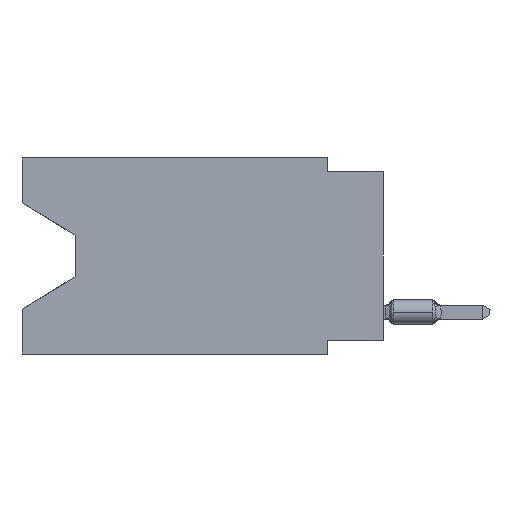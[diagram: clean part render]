
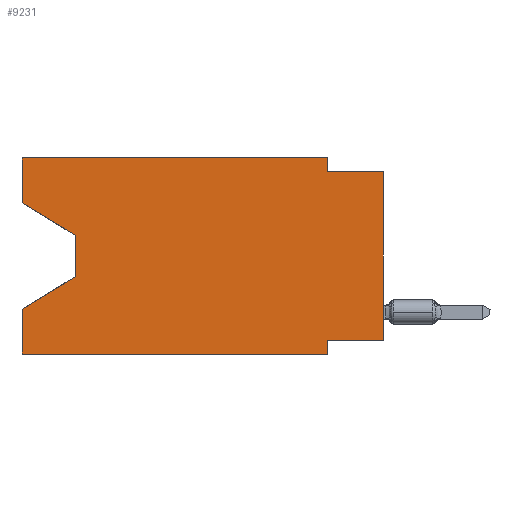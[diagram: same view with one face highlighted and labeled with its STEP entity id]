
A CAD part, left-side view. The second image highlights one B-rep face of the part: STEP entity #9231.
In plain terms, the highlighted planar face has unit normal (-1, 0, 0).
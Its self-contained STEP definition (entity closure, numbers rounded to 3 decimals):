
#89 = DIRECTION ( 'NONE',  ( 0., -0.855, -0.519 ) ) ;
#233 = CARTESIAN_POINT ( 'NONE',  ( 0., 16.383, 0. ) ) ;
#624 = ORIENTED_EDGE ( 'NONE', *, *, #20183, .T. ) ;
#1075 = ORIENTED_EDGE ( 'NONE', *, *, #25123, .T. ) ;
#1154 = CARTESIAN_POINT ( 'NONE',  ( 0., 16.383, 0. ) ) ;
#2207 = EDGE_CURVE ( 'NONE', #17085, #7352, #25438, .T. ) ;
#2250 = EDGE_CURVE ( 'NONE', #11897, #16530, #12424, .T. ) ;
#2312 = CARTESIAN_POINT ( 'NONE',  ( 0., 13.97, -5.385 ) ) ;
#2490 = PLANE ( 'NONE',  #31888 ) ;
#2529 = VECTOR ( 'NONE', #15556, 1000. ) ;
#3040 = EDGE_CURVE ( 'NONE', #7210, #9393, #24989, .T. ) ;
#3140 = VERTEX_POINT ( 'NONE', #23352 ) ;
#3518 = EDGE_CURVE ( 'NONE', #7352, #16530, #30788, .T. ) ;
#3834 = CARTESIAN_POINT ( 'NONE',  ( 0., 0., -8.255 ) ) ;
#4276 = ORIENTED_EDGE ( 'NONE', *, *, #25772, .F. ) ;
#4380 = LINE ( 'NONE', #15227, #20612 ) ;
#4514 = VECTOR ( 'NONE', #32102, 1000. ) ;
#4566 = LINE ( 'NONE', #23581, #4514 ) ;
#4785 = VECTOR ( 'NONE', #17779, 1000. ) ;
#5149 = DIRECTION ( 'NONE',  ( 1., 0., 0. ) ) ;
#5210 = VERTEX_POINT ( 'NONE', #28147 ) ;
#5321 = CARTESIAN_POINT ( 'NONE',  ( 0., 16.383, 0. ) ) ;
#6059 = CARTESIAN_POINT ( 'NONE',  ( 0., 2.54, -0.635 ) ) ;
#6115 = VECTOR ( 'NONE', #89, 1000. ) ;
#6906 = CARTESIAN_POINT ( 'NONE',  ( 0., 2.54, -8.89 ) ) ;
#7210 = VERTEX_POINT ( 'NONE', #2312 ) ;
#7352 = VERTEX_POINT ( 'NONE', #22215 ) ;
#7535 = LINE ( 'NONE', #32271, #6115 ) ;
#7767 = CARTESIAN_POINT ( 'NONE',  ( 0., 0., -0.635 ) ) ;
#8095 = EDGE_CURVE ( 'NONE', #17085, #34707, #4380, .T. ) ;
#8875 = VECTOR ( 'NONE', #14581, 1000. ) ;
#9231 = ADVANCED_FACE ( 'NONE', ( #29511 ), #2490, .F. ) ;
#9393 = VERTEX_POINT ( 'NONE', #30914 ) ;
#9701 = VERTEX_POINT ( 'NONE', #1154 ) ;
#9958 = VECTOR ( 'NONE', #24852, 1000. ) ;
#10152 = DIRECTION ( 'NONE',  ( 0., 0., -1. ) ) ;
#10633 = CARTESIAN_POINT ( 'NONE',  ( 0., 2.54, -8.89 ) ) ;
#10698 = ORIENTED_EDGE ( 'NONE', *, *, #22738, .F. ) ;
#11897 = VERTEX_POINT ( 'NONE', #25189 ) ;
#12424 = LINE ( 'NONE', #33763, #8875 ) ;
#14377 = ORIENTED_EDGE ( 'NONE', *, *, #33634, .F. ) ;
#14581 = DIRECTION ( 'NONE',  ( 0., -1., 0. ) ) ;
#14922 = CARTESIAN_POINT ( 'NONE',  ( 0., 0., -8.255 ) ) ;
#15227 = CARTESIAN_POINT ( 'NONE',  ( 0., 0., 0. ) ) ;
#15247 = ORIENTED_EDGE ( 'NONE', *, *, #3040, .T. ) ;
#15556 = DIRECTION ( 'NONE',  ( 0., 0., 1. ) ) ;
#15677 = LINE ( 'NONE', #24022, #20186 ) ;
#16282 = CARTESIAN_POINT ( 'NONE',  ( 0., 2.54, 0. ) ) ;
#16530 = VERTEX_POINT ( 'NONE', #10633 ) ;
#16658 = LINE ( 'NONE', #21818, #9958 ) ;
#17085 = VERTEX_POINT ( 'NONE', #3834 ) ;
#17779 = DIRECTION ( 'NONE',  ( 0., 0., -1. ) ) ;
#19285 = LINE ( 'NONE', #233, #31623 ) ;
#19436 = EDGE_LOOP ( 'NONE', ( #1075, #624, #15247, #10698, #22197, #28605, #26806, #34884, #4276, #21616, #14377, #19719 ) ) ;
#19719 = ORIENTED_EDGE ( 'NONE', *, *, #29142, .F. ) ;
#20183 = EDGE_CURVE ( 'NONE', #5210, #7210, #15677, .T. ) ;
#20186 = VECTOR ( 'NONE', #10152, 1000. ) ;
#20612 = VECTOR ( 'NONE', #22529, 1000. ) ;
#21587 = DIRECTION ( 'NONE',  ( 0., 0., 1. ) ) ;
#21616 = ORIENTED_EDGE ( 'NONE', *, *, #27350, .F. ) ;
#21818 = CARTESIAN_POINT ( 'NONE',  ( 0., 16.383, 0. ) ) ;
#22197 = ORIENTED_EDGE ( 'NONE', *, *, #2250, .T. ) ;
#22215 = CARTESIAN_POINT ( 'NONE',  ( 0., 2.54, -8.255 ) ) ;
#22529 = DIRECTION ( 'NONE',  ( 0., 0., 1. ) ) ;
#22738 = EDGE_CURVE ( 'NONE', #11897, #9393, #31549, .T. ) ;
#23352 = CARTESIAN_POINT ( 'NONE',  ( 0., 16.383, -2.038 ) ) ;
#23479 = CARTESIAN_POINT ( 'NONE',  ( 0., 0., -0.635 ) ) ;
#23551 = CARTESIAN_POINT ( 'NONE',  ( 0., 16.383, 0. ) ) ;
#23581 = CARTESIAN_POINT ( 'NONE',  ( 0., 2.54, 0. ) ) ;
#24022 = CARTESIAN_POINT ( 'NONE',  ( 0., 13.97, -3.505 ) ) ;
#24852 = DIRECTION ( 'NONE',  ( 0., -1., 0. ) ) ;
#24887 = VECTOR ( 'NONE', #34149, 1000. ) ;
#24989 = LINE ( 'NONE', #28349, #29838 ) ;
#25123 = EDGE_CURVE ( 'NONE', #3140, #5210, #7535, .T. ) ;
#25189 = CARTESIAN_POINT ( 'NONE',  ( 0., 16.383, -8.89 ) ) ;
#25342 = DIRECTION ( 'NONE',  ( 0., 0.855, -0.519 ) ) ;
#25438 = LINE ( 'NONE', #14922, #29298 ) ;
#25772 = EDGE_CURVE ( 'NONE', #35158, #34707, #31471, .T. ) ;
#25777 = DIRECTION ( 'NONE',  ( 0., 1., 0. ) ) ;
#26242 = VERTEX_POINT ( 'NONE', #16282 ) ;
#26806 = ORIENTED_EDGE ( 'NONE', *, *, #2207, .F. ) ;
#26855 = DIRECTION ( 'NONE',  ( 0., 0., -1. ) ) ;
#27350 = EDGE_CURVE ( 'NONE', #26242, #35158, #4566, .T. ) ;
#28147 = CARTESIAN_POINT ( 'NONE',  ( 0., 13.97, -3.505 ) ) ;
#28349 = CARTESIAN_POINT ( 'NONE',  ( 0., 13.97, -5.385 ) ) ;
#28605 = ORIENTED_EDGE ( 'NONE', *, *, #3518, .F. ) ;
#29142 = EDGE_CURVE ( 'NONE', #3140, #9701, #19285, .T. ) ;
#29298 = VECTOR ( 'NONE', #25777, 1000. ) ;
#29511 = FACE_OUTER_BOUND ( 'NONE', #19436, .T. ) ;
#29838 = VECTOR ( 'NONE', #25342, 1000. ) ;
#30788 = LINE ( 'NONE', #6906, #4785 ) ;
#30914 = CARTESIAN_POINT ( 'NONE',  ( 0., 16.383, -6.852 ) ) ;
#31471 = LINE ( 'NONE', #23479, #24887 ) ;
#31549 = LINE ( 'NONE', #23551, #2529 ) ;
#31623 = VECTOR ( 'NONE', #21587, 1000. ) ;
#31888 = AXIS2_PLACEMENT_3D ( 'NONE', #5321, #5149, #26855 ) ;
#32102 = DIRECTION ( 'NONE',  ( 0., 0., -1. ) ) ;
#32271 = CARTESIAN_POINT ( 'NONE',  ( 0., 16.383, -2.038 ) ) ;
#33634 = EDGE_CURVE ( 'NONE', #9701, #26242, #16658, .T. ) ;
#33763 = CARTESIAN_POINT ( 'NONE',  ( 0., 16.383, -8.89 ) ) ;
#34149 = DIRECTION ( 'NONE',  ( 0., -1., 0. ) ) ;
#34707 = VERTEX_POINT ( 'NONE', #7767 ) ;
#34884 = ORIENTED_EDGE ( 'NONE', *, *, #8095, .T. ) ;
#35158 = VERTEX_POINT ( 'NONE', #6059 ) ;
